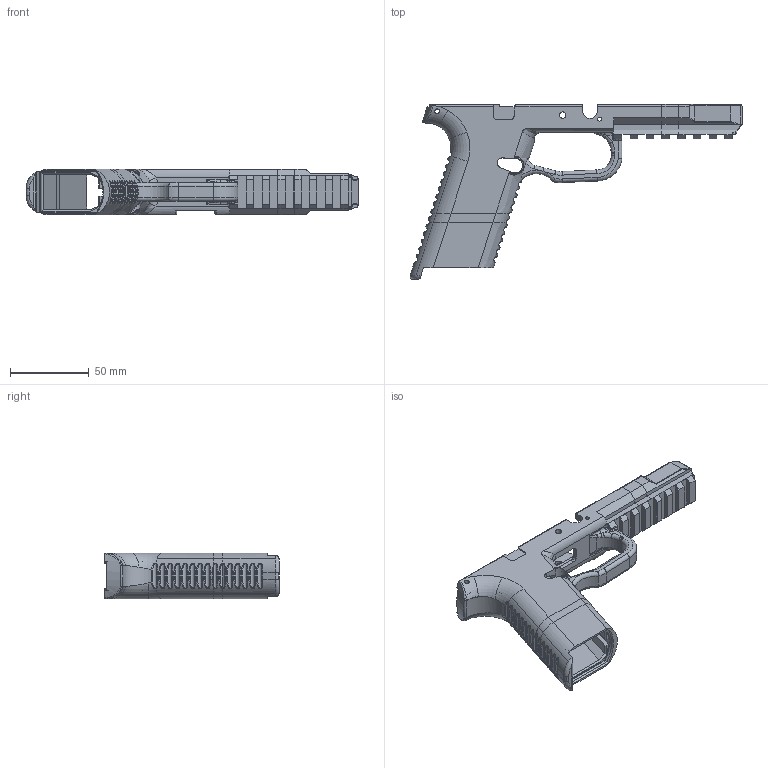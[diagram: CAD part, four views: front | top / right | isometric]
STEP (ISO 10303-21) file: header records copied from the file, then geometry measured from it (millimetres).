
FILE_DESCRIPTION (( 'STEP AP203' ), '1' );
FILE_NAME ('SkinnyGrip Longboi.STEP', '2021-06-01T22:47:40', ( '' ), ( '' ), 'SwSTEP 2.0', 'SolidWorks 2020', '' );
FILE_SCHEMA (( 'CONFIG_CONTROL_DESIGN' ));
Products named in the file (1): SkinnyGrip Longboi
Bounding box: 210.6 x 110.97 x 29 mm (x, y, z)
Volume: 88842.2 mm3; surface area: 51671.4 mm2
Topology: 5 solids, 5 shells, 728 faces, 1986 edges, 1261 vertices
Faces by surface type: plane 298, cylinder 258, bspline 124, torus 38, cone 6, sphere 4
Entity records: 42425 total; most frequent: CARTESIAN_POINT 25202, ORIENTED_EDGE 3960, DIRECTION 3113, EDGE_CURVE 1980, VERTEX_POINT 1261, VECTOR 1075, LINE 1075, AXIS2_PLACEMENT_3D 1019
